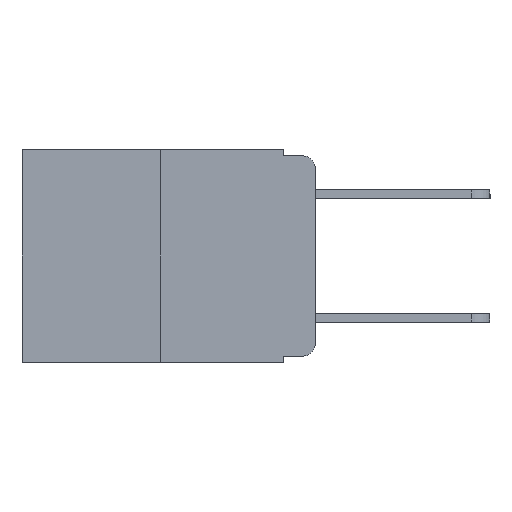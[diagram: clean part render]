
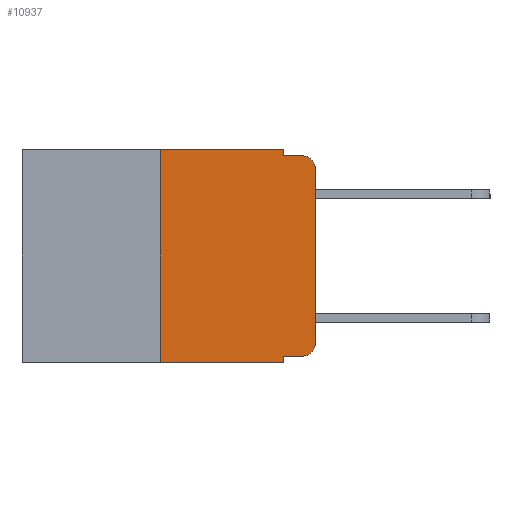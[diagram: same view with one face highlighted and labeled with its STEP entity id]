
A CAD part, left-side view. The second image highlights one B-rep face of the part: STEP entity #10937.
In plain terms, the highlighted planar face has unit normal (-1, 0, 0).
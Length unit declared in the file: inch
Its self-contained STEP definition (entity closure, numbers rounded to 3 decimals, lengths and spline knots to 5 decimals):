
#97 = LINE ( 'NONE', #9981, #9930 ) ;
#133 = VECTOR ( 'NONE', #15086, 39.37008 ) ;
#191 = VERTEX_POINT ( 'NONE', #10272 ) ;
#248 = DIRECTION ( 'NONE',  ( 0., -1., 0. ) ) ;
#264 = EDGE_CURVE ( 'NONE', #14624, #7538, #5691, .T. ) ;
#938 = ORIENTED_EDGE ( 'NONE', *, *, #2253, .T. ) ;
#1215 = ORIENTED_EDGE ( 'NONE', *, *, #264, .T. ) ;
#1415 = CARTESIAN_POINT ( 'NONE',  ( 0., 0.02, -0.01 ) ) ;
#1526 = LINE ( 'NONE', #5633, #14185 ) ;
#1583 = ORIENTED_EDGE ( 'NONE', *, *, #14693, .F. ) ;
#1706 = ORIENTED_EDGE ( 'NONE', *, *, #13278, .F. ) ;
#1923 = ORIENTED_EDGE ( 'NONE', *, *, #12585, .F. ) ;
#1973 = ORIENTED_EDGE ( 'NONE', *, *, #15538, .F. ) ;
#2034 = LINE ( 'NONE', #12980, #14571 ) ;
#2058 = ORIENTED_EDGE ( 'NONE', *, *, #14126, .T. ) ;
#2125 = VERTEX_POINT ( 'NONE', #9080 ) ;
#2141 = VERTEX_POINT ( 'NONE', #9353 ) ;
#2203 = ORIENTED_EDGE ( 'NONE', *, *, #11832, .F. ) ;
#2253 = EDGE_CURVE ( 'NONE', #9053, #14624, #13661, .T. ) ;
#2374 = ORIENTED_EDGE ( 'NONE', *, *, #7968, .T. ) ;
#2446 = ORIENTED_EDGE ( 'NONE', *, *, #6281, .T. ) ;
#2583 = CARTESIAN_POINT ( 'NONE',  ( 0., 0.02, -0.03 ) ) ;
#2860 = DIRECTION ( 'NONE',  ( 0., 0., 1. ) ) ;
#2940 = DIRECTION ( 'NONE',  ( 0., 0., -1. ) ) ;
#3002 = CARTESIAN_POINT ( 'NONE',  ( 0., 0., -0.313 ) ) ;
#3581 = CARTESIAN_POINT ( 'NONE',  ( 0., 0.051, -0.01 ) ) ;
#3663 = DIRECTION ( 'NONE',  ( 0., -1., 0. ) ) ;
#3766 = VERTEX_POINT ( 'NONE', #15294 ) ;
#3911 = CARTESIAN_POINT ( 'NONE',  ( 0., 0.473, 0. ) ) ;
#5249 = DIRECTION ( 'NONE',  ( 1., 0., 0. ) ) ;
#5366 = EDGE_LOOP ( 'NONE', ( #938, #1215, #1583, #1706, #1973, #1923, #2058, #2203, #2374, #2446 ) ) ;
#5464 = CARTESIAN_POINT ( 'NONE',  ( 0., 0.051, 0. ) ) ;
#5633 = CARTESIAN_POINT ( 'NONE',  ( 0., 0.051, 0. ) ) ;
#5639 = AXIS2_PLACEMENT_3D ( 'NONE', #2583, #8027, #10856 ) ;
#5691 = CIRCLE ( 'NONE', #5639, 0.02 ) ;
#6281 = EDGE_CURVE ( 'NONE', #2125, #9053, #10334, .T. ) ;
#6337 = CARTESIAN_POINT ( 'NONE',  ( 0., 0.25, -0.343 ) ) ;
#6888 = LINE ( 'NONE', #5464, #7280 ) ;
#7180 = CARTESIAN_POINT ( 'NONE',  ( 0., 0.02, -0.313 ) ) ;
#7280 = VECTOR ( 'NONE', #12580, 39.37008 ) ;
#7527 = DIRECTION ( 'NONE',  ( 0., -1., 0. ) ) ;
#7538 = VERTEX_POINT ( 'NONE', #1415 ) ;
#7968 = EDGE_CURVE ( 'NONE', #191, #2125, #97, .T. ) ;
#8027 = DIRECTION ( 'NONE',  ( -1., 0., 0. ) ) ;
#8414 = DIRECTION ( 'NONE',  ( 0., 0., -1. ) ) ;
#8501 = DIRECTION ( 'NONE',  ( 0., -1., 0. ) ) ;
#9053 = VERTEX_POINT ( 'NONE', #3002 ) ;
#9080 = CARTESIAN_POINT ( 'NONE',  ( 0., 0.02, -0.333 ) ) ;
#9334 = LINE ( 'NONE', #12953, #14467 ) ;
#9353 = CARTESIAN_POINT ( 'NONE',  ( 0., 0.25, 0. ) ) ;
#9930 = VECTOR ( 'NONE', #3663, 39.37008 ) ;
#9981 = CARTESIAN_POINT ( 'NONE',  ( 0., 0.051, -0.333 ) ) ;
#10154 = LINE ( 'NONE', #15332, #13056 ) ;
#10167 = FACE_OUTER_BOUND ( 'NONE', #5366, .T. ) ;
#10272 = CARTESIAN_POINT ( 'NONE',  ( 0., 0.051, -0.333 ) ) ;
#10334 = CIRCLE ( 'NONE', #15485, 0.02 ) ;
#10704 = CARTESIAN_POINT ( 'NONE',  ( 0., 0.25, 0. ) ) ;
#10776 = VECTOR ( 'NONE', #2860, 39.37008 ) ;
#10818 = VERTEX_POINT ( 'NONE', #6337 ) ;
#10856 = DIRECTION ( 'NONE',  ( 0., 0., -1. ) ) ;
#10937 = ADVANCED_FACE ( 'NONE', ( #10167 ), #11295, .F. ) ;
#11295 = PLANE ( 'NONE',  #14444 ) ;
#11467 = VERTEX_POINT ( 'NONE', #14122 ) ;
#11472 = VERTEX_POINT ( 'NONE', #3581 ) ;
#11832 = EDGE_CURVE ( 'NONE', #191, #11467, #1526, .T. ) ;
#12580 = DIRECTION ( 'NONE',  ( 0., 0., -1. ) ) ;
#12585 = EDGE_CURVE ( 'NONE', #10818, #2141, #13538, .T. ) ;
#12953 = CARTESIAN_POINT ( 'NONE',  ( 0., 0.473, -0.343 ) ) ;
#12980 = CARTESIAN_POINT ( 'NONE',  ( 0., 0.051, -0.01 ) ) ;
#13056 = VECTOR ( 'NONE', #7527, 39.37008 ) ;
#13278 = EDGE_CURVE ( 'NONE', #3766, #11472, #6888, .T. ) ;
#13460 = DIRECTION ( 'NONE',  ( 0., 0., -1. ) ) ;
#13538 = LINE ( 'NONE', #10704, #133 ) ;
#13661 = LINE ( 'NONE', #15873, #10776 ) ;
#13948 = CARTESIAN_POINT ( 'NONE',  ( 0., 0., -0.03 ) ) ;
#14122 = CARTESIAN_POINT ( 'NONE',  ( 0., 0.051, -0.343 ) ) ;
#14126 = EDGE_CURVE ( 'NONE', #10818, #11467, #9334, .T. ) ;
#14185 = VECTOR ( 'NONE', #2940, 39.37008 ) ;
#14444 = AXIS2_PLACEMENT_3D ( 'NONE', #3911, #5249, #13460 ) ;
#14467 = VECTOR ( 'NONE', #248, 39.37008 ) ;
#14571 = VECTOR ( 'NONE', #8501, 39.37008 ) ;
#14624 = VERTEX_POINT ( 'NONE', #13948 ) ;
#14693 = EDGE_CURVE ( 'NONE', #11472, #7538, #2034, .T. ) ;
#15044 = DIRECTION ( 'NONE',  ( -1., 0., 0. ) ) ;
#15086 = DIRECTION ( 'NONE',  ( 0., 0., 1. ) ) ;
#15294 = CARTESIAN_POINT ( 'NONE',  ( 0., 0.051, 0. ) ) ;
#15332 = CARTESIAN_POINT ( 'NONE',  ( 0., 0.473, 0. ) ) ;
#15485 = AXIS2_PLACEMENT_3D ( 'NONE', #7180, #15044, #8414 ) ;
#15538 = EDGE_CURVE ( 'NONE', #2141, #3766, #10154, .T. ) ;
#15873 = CARTESIAN_POINT ( 'NONE',  ( 0., 0., 0. ) ) ;
